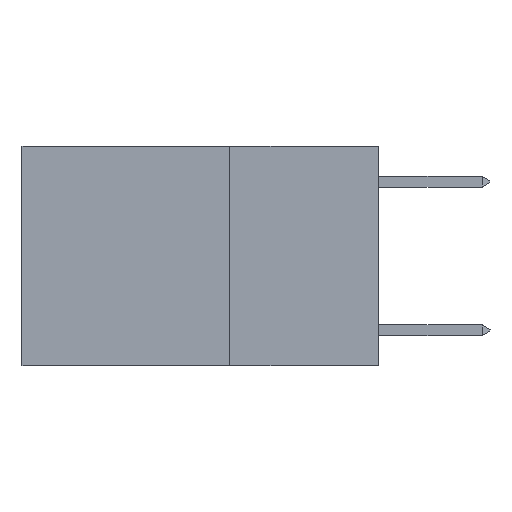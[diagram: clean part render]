
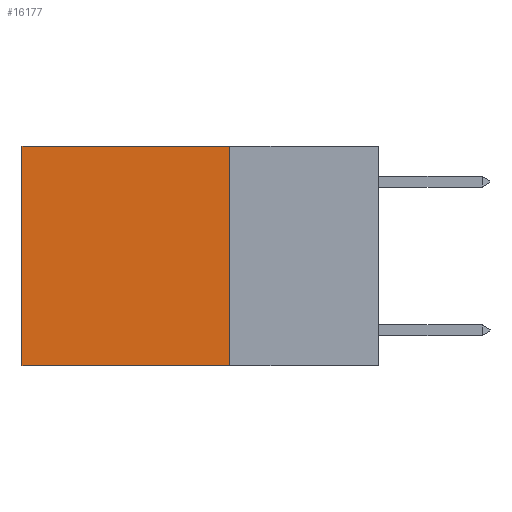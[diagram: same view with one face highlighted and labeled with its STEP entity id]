
A CAD part, left-side view. The second image highlights one B-rep face of the part: STEP entity #16177.
In plain terms, the highlighted planar face has unit normal (-1, 0, 0).
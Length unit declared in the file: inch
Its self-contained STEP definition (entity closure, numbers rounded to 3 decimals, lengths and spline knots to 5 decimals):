
#70 = VECTOR ( 'NONE', #8829, 39.37008 ) ;
#278 = ORIENTED_EDGE ( 'NONE', *, *, #12241, .F. ) ;
#522 = FACE_OUTER_BOUND ( 'NONE', #13051, .T. ) ;
#1655 = VERTEX_POINT ( 'NONE', #7936 ) ;
#2857 = CARTESIAN_POINT ( 'NONE',  ( 0.2625, 0.25, 0. ) ) ;
#3063 = CARTESIAN_POINT ( 'NONE',  ( 0.2625, 0.25, -0.37 ) ) ;
#3860 = DIRECTION ( 'NONE',  ( 0., 1., 0. ) ) ;
#4058 = LINE ( 'NONE', #4438, #70 ) ;
#4215 = VECTOR ( 'NONE', #11630, 39.37008 ) ;
#4438 = CARTESIAN_POINT ( 'NONE',  ( 0.2625, 0.6, 0. ) ) ;
#5845 = VECTOR ( 'NONE', #3860, 39.37008 ) ;
#6824 = AXIS2_PLACEMENT_3D ( 'NONE', #17055, #8495, #18441 ) ;
#7200 = LINE ( 'NONE', #14472, #4215 ) ;
#7331 = DIRECTION ( 'NONE',  ( 0., 1., 0. ) ) ;
#7560 = ORIENTED_EDGE ( 'NONE', *, *, #12244, .T. ) ;
#7936 = CARTESIAN_POINT ( 'NONE',  ( 0.2625, 0.25, 0. ) ) ;
#8377 = ORIENTED_EDGE ( 'NONE', *, *, #17669, .T. ) ;
#8495 = DIRECTION ( 'NONE',  ( 1., 0., 0. ) ) ;
#8829 = DIRECTION ( 'NONE',  ( 0., 0., -1. ) ) ;
#8972 = VERTEX_POINT ( 'NONE', #3063 ) ;
#9845 = CARTESIAN_POINT ( 'NONE',  ( 0.2625, 0.6, 0. ) ) ;
#9903 = ORIENTED_EDGE ( 'NONE', *, *, #17438, .F. ) ;
#10103 = VECTOR ( 'NONE', #7331, 39.37008 ) ;
#10104 = VERTEX_POINT ( 'NONE', #9845 ) ;
#10127 = LINE ( 'NONE', #13994, #5845 ) ;
#11630 = DIRECTION ( 'NONE',  ( 0., 0., -1. ) ) ;
#11967 = CARTESIAN_POINT ( 'NONE',  ( 0.2625, 0.6, -0.37 ) ) ;
#12241 = EDGE_CURVE ( 'NONE', #1655, #8972, #7200, .T. ) ;
#12244 = EDGE_CURVE ( 'NONE', #1655, #10104, #17688, .T. ) ;
#13051 = EDGE_LOOP ( 'NONE', ( #8377, #9903, #278, #7560 ) ) ;
#13994 = CARTESIAN_POINT ( 'NONE',  ( 0.2625, 0.25, -0.37 ) ) ;
#14217 = PLANE ( 'NONE',  #6824 ) ;
#14472 = CARTESIAN_POINT ( 'NONE',  ( 0.2625, 0.25, 0. ) ) ;
#16177 = ADVANCED_FACE ( 'NONE', ( #522 ), #14217, .F. ) ;
#17055 = CARTESIAN_POINT ( 'NONE',  ( 0.2625, 0.25, 0. ) ) ;
#17438 = EDGE_CURVE ( 'NONE', #8972, #18117, #10127, .T. ) ;
#17669 = EDGE_CURVE ( 'NONE', #10104, #18117, #4058, .T. ) ;
#17688 = LINE ( 'NONE', #2857, #10103 ) ;
#18117 = VERTEX_POINT ( 'NONE', #11967 ) ;
#18441 = DIRECTION ( 'NONE',  ( 0., 0., -1. ) ) ;
